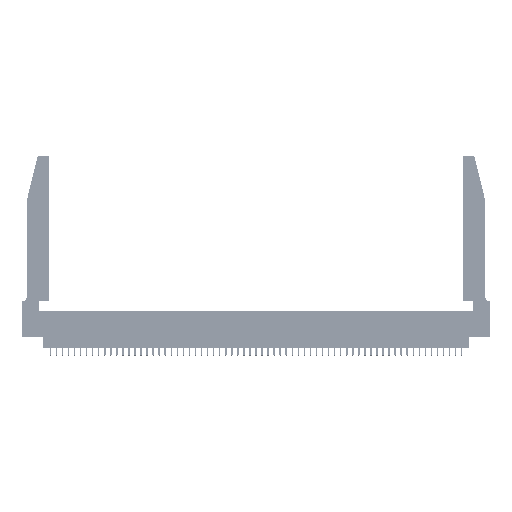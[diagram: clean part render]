
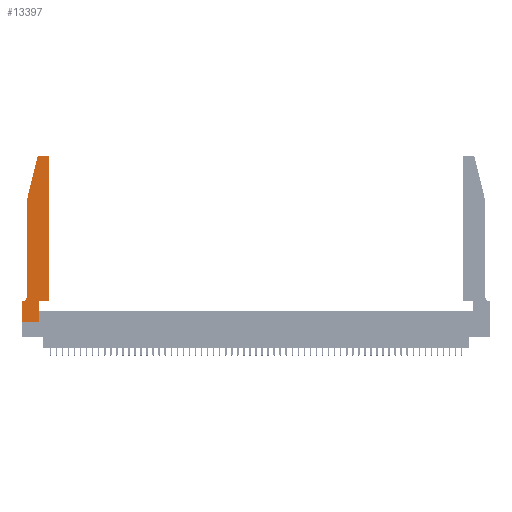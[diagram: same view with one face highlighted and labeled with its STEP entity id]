
A CAD part, top view. The second image highlights one B-rep face of the part: STEP entity #13397.
In plain terms, the highlighted planar face has unit normal (0, 0, 1).
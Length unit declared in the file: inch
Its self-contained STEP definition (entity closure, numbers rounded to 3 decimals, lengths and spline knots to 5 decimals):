
#286 = VERTEX_POINT ( 'NONE', #43495 ) ;
#437 = EDGE_LOOP ( 'NONE', ( #6324, #39326, #4199, #55429, #27688, #44475, #34656, #55046, #23394, #29853, #46912, #32439 ) ) ;
#604 = CARTESIAN_POINT ( 'NONE',  ( 0.2865, 0.35, 0.37 ) ) ;
#687 = CARTESIAN_POINT ( 'NONE',  ( 0.4205, 2.72, 0.37 ) ) ;
#1280 = VECTOR ( 'NONE', #6754, 39.37008 ) ;
#1535 = AXIS2_PLACEMENT_3D ( 'NONE', #3925, #46637, #20963 ) ;
#2092 = CARTESIAN_POINT ( 'NONE',  ( 0.4505, 0.35, 0.37 ) ) ;
#2094 = VECTOR ( 'NONE', #29574, 39.37008 ) ;
#2866 = EDGE_CURVE ( 'NONE', #53779, #51293, #11309, .T. ) ;
#3794 = LINE ( 'NONE', #38749, #9158 ) ;
#3925 = CARTESIAN_POINT ( 'NONE',  ( 0., 0.35, 0.37 ) ) ;
#4199 = ORIENTED_EDGE ( 'NONE', *, *, #52070, .T. ) ;
#5310 = LINE ( 'NONE', #2092, #1280 ) ;
#6146 = CARTESIAN_POINT ( 'NONE',  ( 0.2605, 2.75, 0.37 ) ) ;
#6198 = CARTESIAN_POINT ( 'NONE',  ( 0.0755, 2., 0.37 ) ) ;
#6324 = ORIENTED_EDGE ( 'NONE', *, *, #36816, .T. ) ;
#6387 = AXIS2_PLACEMENT_3D ( 'NONE', #687, #9302, #39254 ) ;
#6754 = DIRECTION ( 'NONE',  ( 1., 0., 0. ) ) ;
#7193 = VECTOR ( 'NONE', #28207, 39.37008 ) ;
#7557 = CARTESIAN_POINT ( 'NONE',  ( 0., 0., 0.37 ) ) ;
#8076 = CARTESIAN_POINT ( 'NONE',  ( 0.25487, 2.72718, 0.37 ) ) ;
#8562 = VERTEX_POINT ( 'NONE', #37728 ) ;
#9158 = VECTOR ( 'NONE', #22254, 39.37008 ) ;
#9253 = VERTEX_POINT ( 'NONE', #50578 ) ;
#9302 = DIRECTION ( 'NONE',  ( 0., 0., 1. ) ) ;
#9678 = CARTESIAN_POINT ( 'NONE',  ( 0.2865, 0., 0.37 ) ) ;
#11309 = CIRCLE ( 'NONE', #47328, 0.03 ) ;
#12113 = DIRECTION ( 'NONE',  ( 1., 0., 0. ) ) ;
#13397 = ADVANCED_FACE ( 'NONE', ( #53227 ), #16630, .T. ) ;
#14111 = AXIS2_PLACEMENT_3D ( 'NONE', #30115, #52037, #39296 ) ;
#15136 = VERTEX_POINT ( 'NONE', #37648 ) ;
#15216 = LINE ( 'NONE', #6146, #7193 ) ;
#15349 = LINE ( 'NONE', #24455, #38176 ) ;
#15402 = CARTESIAN_POINT ( 'NONE',  ( 0.2865, 0.35, 0.37 ) ) ;
#16630 = PLANE ( 'NONE',  #1535 ) ;
#17282 = VERTEX_POINT ( 'NONE', #6198 ) ;
#17788 = VERTEX_POINT ( 'NONE', #9678 ) ;
#18896 = CARTESIAN_POINT ( 'NONE',  ( 0.284, 2.75, 0.37 ) ) ;
#19201 = DIRECTION ( 'NONE',  ( 0., 1., 0. ) ) ;
#20066 = CIRCLE ( 'NONE', #14111, 0.07 ) ;
#20647 = EDGE_CURVE ( 'NONE', #24370, #17788, #21526, .T. ) ;
#20963 = DIRECTION ( 'NONE',  ( 1., 0., 0. ) ) ;
#21526 = LINE ( 'NONE', #54112, #24855 ) ;
#21910 = EDGE_CURVE ( 'NONE', #17788, #22238, #34131, .T. ) ;
#22238 = VERTEX_POINT ( 'NONE', #604 ) ;
#22254 = DIRECTION ( 'NONE',  ( 0., -1., 0. ) ) ;
#22735 = DIRECTION ( 'NONE',  ( -0.239, -0.971, 0. ) ) ;
#23303 = CARTESIAN_POINT ( 'NONE',  ( 0.4505, 0.35, 0.37 ) ) ;
#23394 = ORIENTED_EDGE ( 'NONE', *, *, #21910, .T. ) ;
#24370 = VERTEX_POINT ( 'NONE', #7557 ) ;
#24455 = CARTESIAN_POINT ( 'NONE',  ( 0.4505, 0.35, 0.37 ) ) ;
#24855 = VECTOR ( 'NONE', #36734, 39.37008 ) ;
#25082 = CARTESIAN_POINT ( 'NONE',  ( 0.0755, 0.35, 0.37 ) ) ;
#25583 = CARTESIAN_POINT ( 'NONE',  ( 0.284, 2.72, 0.37 ) ) ;
#25809 = DIRECTION ( 'NONE',  ( 0., -1., 0. ) ) ;
#26807 = CIRCLE ( 'NONE', #6387, 0.03 ) ;
#27688 = ORIENTED_EDGE ( 'NONE', *, *, #39603, .T. ) ;
#27901 = LINE ( 'NONE', #31731, #28553 ) ;
#28207 = DIRECTION ( 'NONE',  ( -1., 0., 0. ) ) ;
#28553 = VECTOR ( 'NONE', #22735, 39.37008 ) ;
#29019 = VERTEX_POINT ( 'NONE', #23303 ) ;
#29574 = DIRECTION ( 'NONE',  ( -1., 0., 0. ) ) ;
#29853 = ORIENTED_EDGE ( 'NONE', *, *, #31635, .T. ) ;
#29892 = DIRECTION ( 'NONE',  ( 0., 0., 1. ) ) ;
#30046 = EDGE_CURVE ( 'NONE', #286, #15136, #48278, .T. ) ;
#30084 = VECTOR ( 'NONE', #25809, 39.37008 ) ;
#30115 = CARTESIAN_POINT ( 'NONE',  ( 0.0055, 0.42, 0.37 ) ) ;
#30723 = EDGE_CURVE ( 'NONE', #9253, #8562, #26807, .T. ) ;
#31635 = EDGE_CURVE ( 'NONE', #22238, #29019, #5310, .T. ) ;
#31731 = CARTESIAN_POINT ( 'NONE',  ( 0.0755, 2., 0.37 ) ) ;
#32439 = ORIENTED_EDGE ( 'NONE', *, *, #30723, .T. ) ;
#34131 = LINE ( 'NONE', #15402, #46864 ) ;
#34656 = ORIENTED_EDGE ( 'NONE', *, *, #51311, .T. ) ;
#34839 = CARTESIAN_POINT ( 'NONE',  ( 0.0755, 2., 0.37 ) ) ;
#36734 = DIRECTION ( 'NONE',  ( 1., 0., 0. ) ) ;
#36816 = EDGE_CURVE ( 'NONE', #8562, #53779, #15216, .T. ) ;
#37648 = CARTESIAN_POINT ( 'NONE',  ( 0., 0.35, 0.37 ) ) ;
#37728 = CARTESIAN_POINT ( 'NONE',  ( 0.4205, 2.75, 0.37 ) ) ;
#38176 = VECTOR ( 'NONE', #46394, 39.37008 ) ;
#38749 = CARTESIAN_POINT ( 'NONE',  ( 0., 0., 0.37 ) ) ;
#39254 = DIRECTION ( 'NONE',  ( 1., 0., 0. ) ) ;
#39296 = DIRECTION ( 'NONE',  ( -1., 0., 0. ) ) ;
#39326 = ORIENTED_EDGE ( 'NONE', *, *, #2866, .T. ) ;
#39603 = EDGE_CURVE ( 'NONE', #47108, #286, #20066, .T. ) ;
#43495 = CARTESIAN_POINT ( 'NONE',  ( 0.0055, 0.35, 0.37 ) ) ;
#44475 = ORIENTED_EDGE ( 'NONE', *, *, #30046, .T. ) ;
#46394 = DIRECTION ( 'NONE',  ( 0., 1., 0. ) ) ;
#46637 = DIRECTION ( 'NONE',  ( 0., 0., 1. ) ) ;
#46864 = VECTOR ( 'NONE', #19201, 39.37008 ) ;
#46912 = ORIENTED_EDGE ( 'NONE', *, *, #49695, .T. ) ;
#47108 = VERTEX_POINT ( 'NONE', #48344 ) ;
#47328 = AXIS2_PLACEMENT_3D ( 'NONE', #25583, #29892, #12113 ) ;
#48278 = LINE ( 'NONE', #25082, #2094 ) ;
#48344 = CARTESIAN_POINT ( 'NONE',  ( 0.0755, 0.42, 0.37 ) ) ;
#49695 = EDGE_CURVE ( 'NONE', #29019, #9253, #15349, .T. ) ;
#50578 = CARTESIAN_POINT ( 'NONE',  ( 0.4505, 2.72, 0.37 ) ) ;
#51293 = VERTEX_POINT ( 'NONE', #8076 ) ;
#51311 = EDGE_CURVE ( 'NONE', #15136, #24370, #3794, .T. ) ;
#51564 = LINE ( 'NONE', #34839, #30084 ) ;
#52037 = DIRECTION ( 'NONE',  ( 0., 0., -1. ) ) ;
#52070 = EDGE_CURVE ( 'NONE', #51293, #17282, #27901, .T. ) ;
#53227 = FACE_OUTER_BOUND ( 'NONE', #437, .T. ) ;
#53487 = EDGE_CURVE ( 'NONE', #17282, #47108, #51564, .T. ) ;
#53779 = VERTEX_POINT ( 'NONE', #18896 ) ;
#54112 = CARTESIAN_POINT ( 'NONE',  ( 0., 0., 0.37 ) ) ;
#55046 = ORIENTED_EDGE ( 'NONE', *, *, #20647, .T. ) ;
#55429 = ORIENTED_EDGE ( 'NONE', *, *, #53487, .T. ) ;
